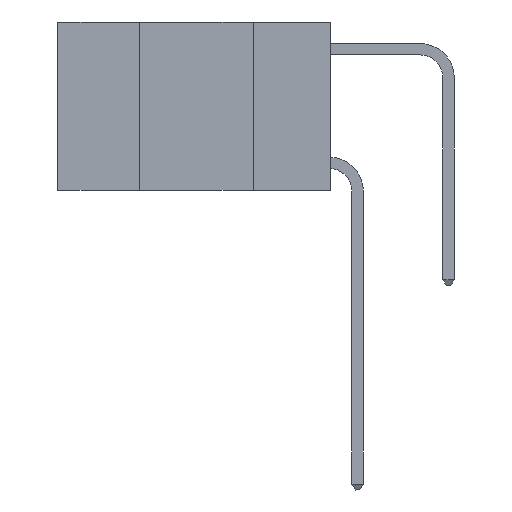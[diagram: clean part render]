
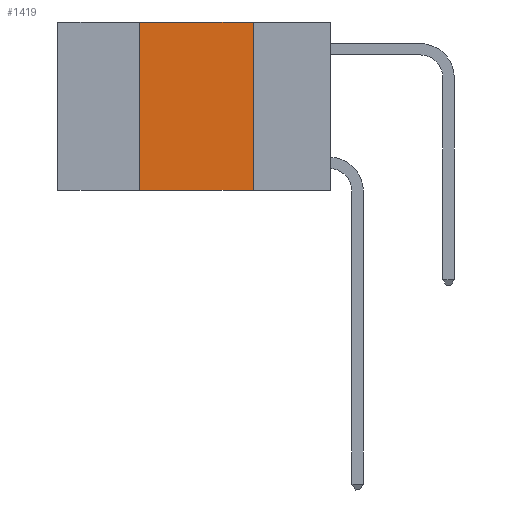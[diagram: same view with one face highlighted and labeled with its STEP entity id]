
A CAD part, left-side view. The second image highlights one B-rep face of the part: STEP entity #1419.
In plain terms, the highlighted planar face has unit normal (-1, 0, 0).
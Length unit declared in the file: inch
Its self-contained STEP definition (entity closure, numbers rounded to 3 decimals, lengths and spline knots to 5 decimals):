
#777 = VECTOR ( 'NONE', #12825, 39.37008 ) ;
#1383 = VERTEX_POINT ( 'NONE', #12635 ) ;
#1419 = ADVANCED_FACE ( 'NONE', ( #13443 ), #12434, .F. ) ;
#1733 = EDGE_LOOP ( 'NONE', ( #7757, #7718, #11888, #9568 ) ) ;
#2115 = CARTESIAN_POINT ( 'NONE',  ( 0., 0.17, 0. ) ) ;
#2175 = CARTESIAN_POINT ( 'NONE',  ( 0., 0.6, 0. ) ) ;
#2450 = EDGE_CURVE ( 'NONE', #3829, #8050, #6104, .T. ) ;
#2926 = DIRECTION ( 'NONE',  ( 0., -1., 0. ) ) ;
#3153 = VECTOR ( 'NONE', #2926, 39.37008 ) ;
#3247 = DIRECTION ( 'NONE',  ( 0., 0., -1. ) ) ;
#3291 = EDGE_CURVE ( 'NONE', #5122, #1383, #12761, .T. ) ;
#3829 = VERTEX_POINT ( 'NONE', #6881 ) ;
#4879 = EDGE_CURVE ( 'NONE', #8050, #1383, #11422, .T. ) ;
#5122 = VERTEX_POINT ( 'NONE', #9934 ) ;
#5235 = LINE ( 'NONE', #7269, #5703 ) ;
#5620 = CARTESIAN_POINT ( 'NONE',  ( 0., 0.6, -0.37 ) ) ;
#5703 = VECTOR ( 'NONE', #7479, 39.37008 ) ;
#6104 = LINE ( 'NONE', #10147, #3153 ) ;
#6228 = DIRECTION ( 'NONE',  ( 0., 0., -1. ) ) ;
#6881 = CARTESIAN_POINT ( 'NONE',  ( 0., 0.42, 0. ) ) ;
#7269 = CARTESIAN_POINT ( 'NONE',  ( 0., 0.42, 0. ) ) ;
#7479 = DIRECTION ( 'NONE',  ( 0., 0., 1. ) ) ;
#7718 = ORIENTED_EDGE ( 'NONE', *, *, #2450, .F. ) ;
#7757 = ORIENTED_EDGE ( 'NONE', *, *, #4879, .F. ) ;
#8002 = CARTESIAN_POINT ( 'NONE',  ( 0., 0.17, 0. ) ) ;
#8050 = VERTEX_POINT ( 'NONE', #8002 ) ;
#9568 = ORIENTED_EDGE ( 'NONE', *, *, #3291, .T. ) ;
#9934 = CARTESIAN_POINT ( 'NONE',  ( 0., 0.42, -0.37 ) ) ;
#10147 = CARTESIAN_POINT ( 'NONE',  ( 0., 0.6, 0. ) ) ;
#11176 = AXIS2_PLACEMENT_3D ( 'NONE', #2175, #11426, #3247 ) ;
#11202 = EDGE_CURVE ( 'NONE', #5122, #3829, #5235, .T. ) ;
#11422 = LINE ( 'NONE', #2115, #13250 ) ;
#11426 = DIRECTION ( 'NONE',  ( 1., 0., 0. ) ) ;
#11888 = ORIENTED_EDGE ( 'NONE', *, *, #11202, .F. ) ;
#12434 = PLANE ( 'NONE',  #11176 ) ;
#12635 = CARTESIAN_POINT ( 'NONE',  ( 0., 0.17, -0.37 ) ) ;
#12761 = LINE ( 'NONE', #5620, #777 ) ;
#12825 = DIRECTION ( 'NONE',  ( 0., -1., 0. ) ) ;
#13250 = VECTOR ( 'NONE', #6228, 39.37008 ) ;
#13443 = FACE_OUTER_BOUND ( 'NONE', #1733, .T. ) ;
